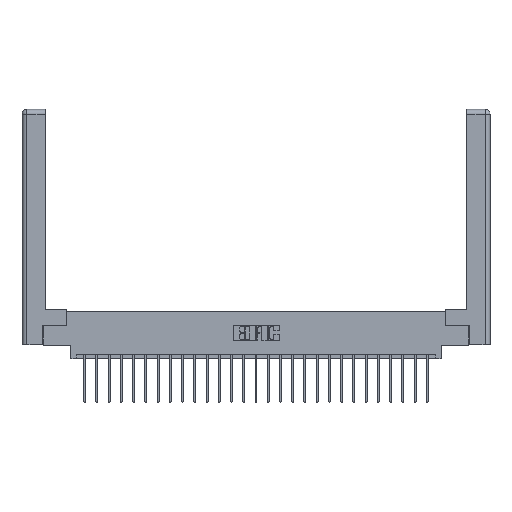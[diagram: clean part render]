
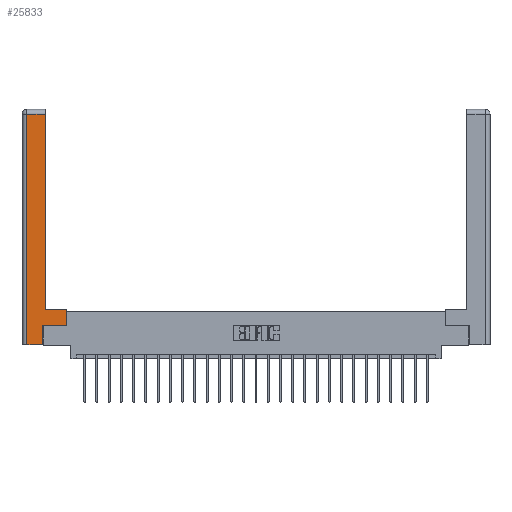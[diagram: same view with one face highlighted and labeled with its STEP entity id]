
A CAD part, top view. The second image highlights one B-rep face of the part: STEP entity #25833.
In plain terms, the highlighted planar face has unit normal (0, 0, 1).
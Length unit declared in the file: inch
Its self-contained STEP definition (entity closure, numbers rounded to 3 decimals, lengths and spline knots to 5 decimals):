
#136 = CARTESIAN_POINT ( 'NONE',  ( 0., 0., 0. ) ) ;
#394 = FACE_OUTER_BOUND ( 'NONE', #20719, .T. ) ;
#404 = EDGE_CURVE ( 'NONE', #14520, #2661, #6956, .T. ) ;
#760 = CARTESIAN_POINT ( 'NONE',  ( 0.0615, 0., 0. ) ) ;
#1142 = DIRECTION ( 'NONE',  ( -1., 0., 0. ) ) ;
#1150 = VECTOR ( 'NONE', #1142, 39.37008 ) ;
#1296 = ORIENTED_EDGE ( 'NONE', *, *, #404, .T. ) ;
#1398 = VECTOR ( 'NONE', #18282, 39.37008 ) ;
#1416 = CARTESIAN_POINT ( 'NONE',  ( 0.565, 0.45, 0. ) ) ;
#1508 = VECTOR ( 'NONE', #16873, 39.37008 ) ;
#1691 = LINE ( 'NONE', #1747, #23277 ) ;
#1747 = CARTESIAN_POINT ( 'NONE',  ( 0.265, 0., 0. ) ) ;
#2096 = CARTESIAN_POINT ( 'NONE',  ( 0.265, 0.245, 0. ) ) ;
#2661 = VERTEX_POINT ( 'NONE', #14880 ) ;
#2759 = CARTESIAN_POINT ( 'NONE',  ( 0.295, 2.94, 0. ) ) ;
#2992 = LINE ( 'NONE', #22449, #6248 ) ;
#3200 = LINE ( 'NONE', #11142, #24763 ) ;
#5714 = VERTEX_POINT ( 'NONE', #19608 ) ;
#6214 = DIRECTION ( 'NONE',  ( 0., 0., -1. ) ) ;
#6248 = VECTOR ( 'NONE', #24536, 39.37008 ) ;
#6322 = EDGE_CURVE ( 'NONE', #2661, #7834, #1691, .T. ) ;
#6726 = CARTESIAN_POINT ( 'NONE',  ( 0.565, 0.245, 0. ) ) ;
#6956 = LINE ( 'NONE', #760, #19380 ) ;
#7046 = LINE ( 'NONE', #10550, #1508 ) ;
#7664 = CARTESIAN_POINT ( 'NONE',  ( 0.0615, 2.94, 0. ) ) ;
#7834 = VERTEX_POINT ( 'NONE', #26825 ) ;
#8575 = VERTEX_POINT ( 'NONE', #6726 ) ;
#9739 = CARTESIAN_POINT ( 'NONE',  ( 0.0615, 2.94, 0. ) ) ;
#10204 = ORIENTED_EDGE ( 'NONE', *, *, #6322, .T. ) ;
#10278 = EDGE_CURVE ( 'NONE', #23927, #5714, #7046, .T. ) ;
#10541 = ORIENTED_EDGE ( 'NONE', *, *, #10278, .T. ) ;
#10550 = CARTESIAN_POINT ( 'NONE',  ( 0.295, 0.45, 0. ) ) ;
#11127 = DIRECTION ( 'NONE',  ( 0., -1., 0. ) ) ;
#11142 = CARTESIAN_POINT ( 'NONE',  ( 0.565, 0.245, 0. ) ) ;
#11712 = PLANE ( 'NONE',  #23433 ) ;
#12026 = ORIENTED_EDGE ( 'NONE', *, *, #16761, .T. ) ;
#12168 = CARTESIAN_POINT ( 'NONE',  ( 0.565, 0.45, 0. ) ) ;
#12321 = DIRECTION ( 'NONE',  ( 0., 1., 0. ) ) ;
#13109 = DIRECTION ( 'NONE',  ( 1., 0., 0. ) ) ;
#14520 = VERTEX_POINT ( 'NONE', #9739 ) ;
#14880 = CARTESIAN_POINT ( 'NONE',  ( 0.0615, 0., 0. ) ) ;
#14990 = VERTEX_POINT ( 'NONE', #2759 ) ;
#16757 = VECTOR ( 'NONE', #12321, 39.37008 ) ;
#16761 = EDGE_CURVE ( 'NONE', #7834, #26018, #18375, .T. ) ;
#16873 = DIRECTION ( 'NONE',  ( -1., 0., 0. ) ) ;
#17896 = ORIENTED_EDGE ( 'NONE', *, *, #24497, .T. ) ;
#18282 = DIRECTION ( 'NONE',  ( 0., 1., 0. ) ) ;
#18353 = LINE ( 'NONE', #1416, #1398 ) ;
#18375 = LINE ( 'NONE', #2096, #16757 ) ;
#18736 = DIRECTION ( 'NONE',  ( -1., 0., 0. ) ) ;
#19191 = ORIENTED_EDGE ( 'NONE', *, *, #21316, .T. ) ;
#19380 = VECTOR ( 'NONE', #11127, 39.37008 ) ;
#19608 = CARTESIAN_POINT ( 'NONE',  ( 0.295, 0.45, 0. ) ) ;
#20089 = ORIENTED_EDGE ( 'NONE', *, *, #22401, .T. ) ;
#20651 = ORIENTED_EDGE ( 'NONE', *, *, #25249, .T. ) ;
#20719 = EDGE_LOOP ( 'NONE', ( #19191, #17896, #1296, #10204, #12026, #20089, #20651, #10541 ) ) ;
#21316 = EDGE_CURVE ( 'NONE', #5714, #14990, #2992, .T. ) ;
#22401 = EDGE_CURVE ( 'NONE', #26018, #8575, #3200, .T. ) ;
#22449 = CARTESIAN_POINT ( 'NONE',  ( 0.295, 3., 0. ) ) ;
#22490 = DIRECTION ( 'NONE',  ( 1., 0., 0. ) ) ;
#23277 = VECTOR ( 'NONE', #22490, 39.37008 ) ;
#23355 = LINE ( 'NONE', #7664, #1150 ) ;
#23433 = AXIS2_PLACEMENT_3D ( 'NONE', #136, #6214, #18736 ) ;
#23927 = VERTEX_POINT ( 'NONE', #12168 ) ;
#24497 = EDGE_CURVE ( 'NONE', #14990, #14520, #23355, .T. ) ;
#24536 = DIRECTION ( 'NONE',  ( 0., 1., 0. ) ) ;
#24763 = VECTOR ( 'NONE', #13109, 39.37008 ) ;
#25249 = EDGE_CURVE ( 'NONE', #8575, #23927, #18353, .T. ) ;
#25833 = ADVANCED_FACE ( 'NONE', ( #394 ), #11712, .F. ) ;
#26018 = VERTEX_POINT ( 'NONE', #26444 ) ;
#26444 = CARTESIAN_POINT ( 'NONE',  ( 0.265, 0.245, 0. ) ) ;
#26825 = CARTESIAN_POINT ( 'NONE',  ( 0.265, 0., 0. ) ) ;
